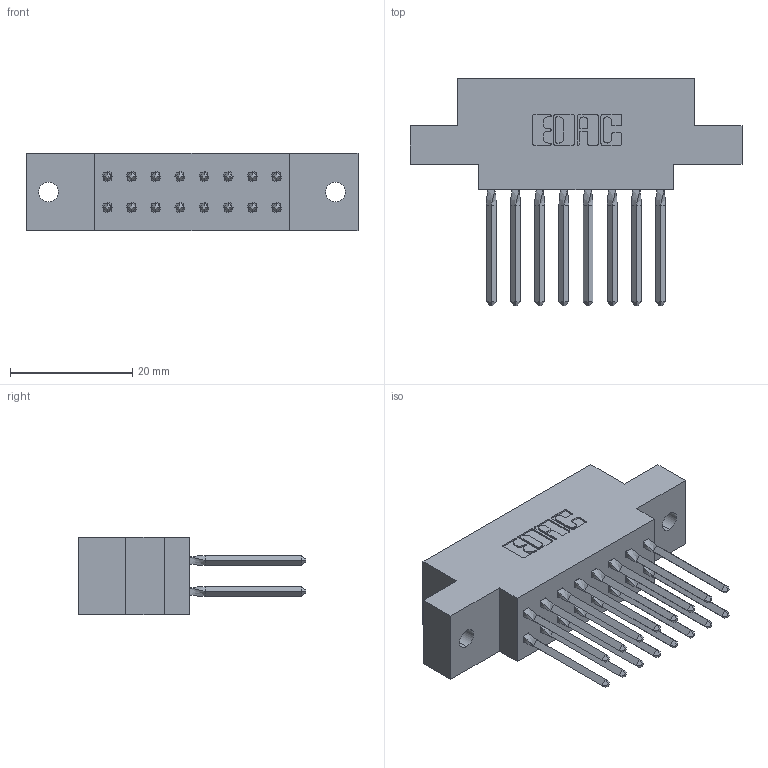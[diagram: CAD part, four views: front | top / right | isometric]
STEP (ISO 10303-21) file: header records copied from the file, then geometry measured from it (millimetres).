
FILE_DESCRIPTION (( 'STEP AP203' ), '1' );
FILE_NAME ('317-016-540-802.STEP', '2020-02-27T15:19:43', ( '' ), ( '' ), 'SwSTEP 2.0', 'SolidWorks 2016', '' );
FILE_SCHEMA (( 'CONFIG_CONTROL_DESIGN' ));
Length unit declared in the file: inch
Products named in the file (3): 317 Part_.144 Dia; 317-016-540-802; 317-290-001_540
Assembly tree (17 placements, depth 2):
  317-016-540-802
    317 Part_.144 Dia
    317-290-001_540  x16
Bounding box: 54.41 x 37.34 x 12.7 mm (x, y, z)
Volume: 7944.9 mm3; surface area: 10297.2 mm2
Topology: 17 solids, 17 shells, 1526 faces, 4227 edges, 2726 vertices
Faces by surface type: plane 1226, cylinder 236, bspline 64
Entity records: 16310 total; most frequent: CARTESIAN_POINT 3255, ORIENTED_EDGE 2754, DIRECTION 2303, EDGE_CURVE 1377, VECTOR 1121, LINE 1121, VERTEX_POINT 911, AXIS2_PLACEMENT_3D 591
